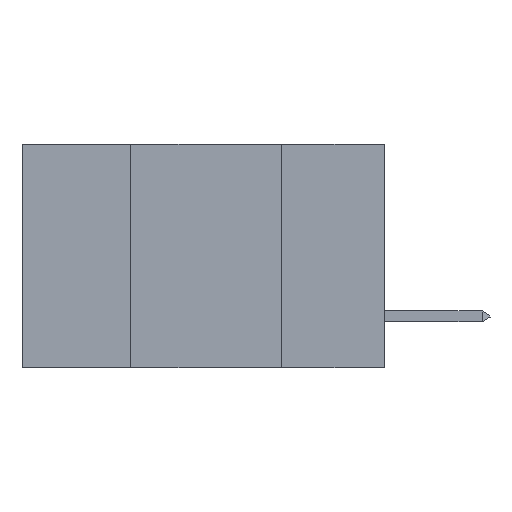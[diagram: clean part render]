
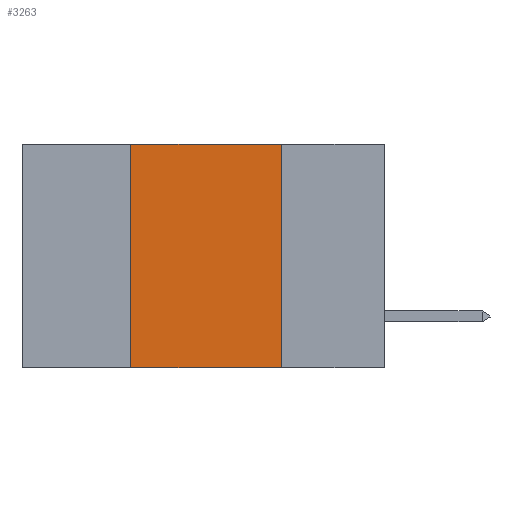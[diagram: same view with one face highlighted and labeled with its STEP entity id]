
A CAD part, left-side view. The second image highlights one B-rep face of the part: STEP entity #3263.
In plain terms, the highlighted planar face has unit normal (-1, 0, 0).
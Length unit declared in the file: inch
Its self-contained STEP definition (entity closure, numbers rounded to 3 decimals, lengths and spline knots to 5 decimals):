
#46 = DIRECTION ( 'NONE',  ( 1., 0., 0. ) ) ;
#397 = DIRECTION ( 'NONE',  ( 0., 0., 1. ) ) ;
#503 = LINE ( 'NONE', #11668, #5600 ) ;
#1015 = CARTESIAN_POINT ( 'NONE',  ( 0., 0.6, -0.37 ) ) ;
#1584 = ORIENTED_EDGE ( 'NONE', *, *, #3360, .T. ) ;
#1732 = FACE_OUTER_BOUND ( 'NONE', #2048, .T. ) ;
#1982 = DIRECTION ( 'NONE',  ( 0., -1., 0. ) ) ;
#2048 = EDGE_LOOP ( 'NONE', ( #3071, #10845, #6393, #1584 ) ) ;
#2594 = DIRECTION ( 'NONE',  ( 0., -1., 0. ) ) ;
#2628 = AXIS2_PLACEMENT_3D ( 'NONE', #9297, #46, #3783 ) ;
#3071 = ORIENTED_EDGE ( 'NONE', *, *, #5352, .F. ) ;
#3079 = CARTESIAN_POINT ( 'NONE',  ( 0., 0.42, -0.37 ) ) ;
#3263 = ADVANCED_FACE ( 'NONE', ( #1732 ), #8341, .F. ) ;
#3340 = VERTEX_POINT ( 'NONE', #10410 ) ;
#3360 = EDGE_CURVE ( 'NONE', #8842, #3340, #3620, .T. ) ;
#3620 = LINE ( 'NONE', #1015, #8250 ) ;
#3783 = DIRECTION ( 'NONE',  ( 0., 0., -1. ) ) ;
#4077 = EDGE_CURVE ( 'NONE', #6998, #11830, #6941, .T. ) ;
#5352 = EDGE_CURVE ( 'NONE', #11830, #3340, #7359, .T. ) ;
#5600 = VECTOR ( 'NONE', #397, 39.37008 ) ;
#5715 = CARTESIAN_POINT ( 'NONE',  ( 0., 0.17, 0. ) ) ;
#6393 = ORIENTED_EDGE ( 'NONE', *, *, #11470, .F. ) ;
#6924 = DIRECTION ( 'NONE',  ( 0., 0., -1. ) ) ;
#6941 = LINE ( 'NONE', #12039, #11482 ) ;
#6998 = VERTEX_POINT ( 'NONE', #8442 ) ;
#7359 = LINE ( 'NONE', #7801, #10159 ) ;
#7801 = CARTESIAN_POINT ( 'NONE',  ( 0., 0.17, 0. ) ) ;
#8250 = VECTOR ( 'NONE', #1982, 39.37008 ) ;
#8341 = PLANE ( 'NONE',  #2628 ) ;
#8442 = CARTESIAN_POINT ( 'NONE',  ( 0., 0.42, 0. ) ) ;
#8842 = VERTEX_POINT ( 'NONE', #3079 ) ;
#9297 = CARTESIAN_POINT ( 'NONE',  ( 0., 0.6, 0. ) ) ;
#10159 = VECTOR ( 'NONE', #6924, 39.37008 ) ;
#10410 = CARTESIAN_POINT ( 'NONE',  ( 0., 0.17, -0.37 ) ) ;
#10845 = ORIENTED_EDGE ( 'NONE', *, *, #4077, .F. ) ;
#11470 = EDGE_CURVE ( 'NONE', #8842, #6998, #503, .T. ) ;
#11482 = VECTOR ( 'NONE', #2594, 39.37008 ) ;
#11668 = CARTESIAN_POINT ( 'NONE',  ( 0., 0.42, 0. ) ) ;
#11830 = VERTEX_POINT ( 'NONE', #5715 ) ;
#12039 = CARTESIAN_POINT ( 'NONE',  ( 0., 0.6, 0. ) ) ;
